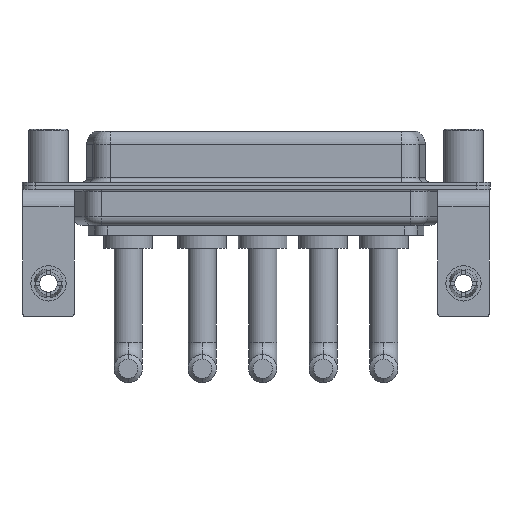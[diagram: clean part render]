
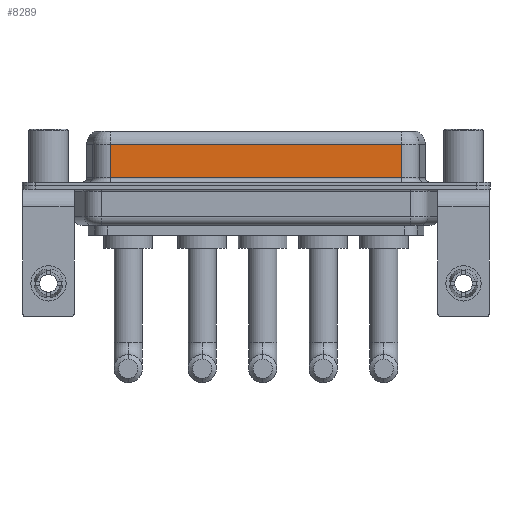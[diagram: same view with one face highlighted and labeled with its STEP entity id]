
A CAD part, front view. The second image highlights one B-rep face of the part: STEP entity #8289.
In plain terms, the highlighted planar face has unit normal (0, -1, 0).
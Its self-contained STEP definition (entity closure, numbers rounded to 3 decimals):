
#295 = VECTOR ( 'NONE', #5341, 1000. ) ;
#356 = CARTESIAN_POINT ( 'NONE',  ( 40.037, -3.95, 4.65 ) ) ;
#391 = PLANE ( 'NONE',  #2152 ) ;
#1579 = LINE ( 'NONE', #356, #295 ) ;
#1739 = ORIENTED_EDGE ( 'NONE', *, *, #10277, .T. ) ;
#2152 = AXIS2_PLACEMENT_3D ( 'NONE', #9179, #5371, #11518 ) ;
#2811 = CARTESIAN_POINT ( 'NONE',  ( 7.013, -3.95, 6.4 ) ) ;
#3545 = DIRECTION ( 'NONE',  ( 0., 0., -1. ) ) ;
#5341 = DIRECTION ( 'NONE',  ( -1., 0., 0. ) ) ;
#5371 = DIRECTION ( 'NONE',  ( 0., 1., 0. ) ) ;
#5410 = CARTESIAN_POINT ( 'NONE',  ( 40.037, -3.95, 0.9 ) ) ;
#5610 = VERTEX_POINT ( 'NONE', #8676 ) ;
#5750 = ORIENTED_EDGE ( 'NONE', *, *, #9745, .T. ) ;
#5841 = LINE ( 'NONE', #8318, #9047 ) ;
#6472 = VECTOR ( 'NONE', #12960, 1000. ) ;
#7248 = CARTESIAN_POINT ( 'NONE',  ( 7.013, -3.95, 0.9 ) ) ;
#7345 = VERTEX_POINT ( 'NONE', #7248 ) ;
#7417 = EDGE_CURVE ( 'NONE', #7345, #12870, #5841, .T. ) ;
#7426 = LINE ( 'NONE', #8497, #13387 ) ;
#7943 = ORIENTED_EDGE ( 'NONE', *, *, #7417, .T. ) ;
#7944 = FACE_OUTER_BOUND ( 'NONE', #11529, .T. ) ;
#8289 = ADVANCED_FACE ( 'NONE', ( #7944 ), #391, .F. ) ;
#8318 = CARTESIAN_POINT ( 'NONE',  ( 40.037, -3.95, 0.9 ) ) ;
#8497 = CARTESIAN_POINT ( 'NONE',  ( 40.037, -3.95, 6.4 ) ) ;
#8676 = CARTESIAN_POINT ( 'NONE',  ( 7.013, -3.95, 4.65 ) ) ;
#9047 = VECTOR ( 'NONE', #11063, 1000. ) ;
#9179 = CARTESIAN_POINT ( 'NONE',  ( 40.037, -3.95, 6.4 ) ) ;
#9745 = EDGE_CURVE ( 'NONE', #5610, #7345, #14123, .T. ) ;
#10277 = EDGE_CURVE ( 'NONE', #13058, #5610, #1579, .T. ) ;
#11063 = DIRECTION ( 'NONE',  ( 1., 0., 0. ) ) ;
#11518 = DIRECTION ( 'NONE',  ( 0., 0., 1. ) ) ;
#11529 = EDGE_LOOP ( 'NONE', ( #16095, #1739, #5750, #7943 ) ) ;
#12561 = EDGE_CURVE ( 'NONE', #13058, #12870, #7426, .T. ) ;
#12870 = VERTEX_POINT ( 'NONE', #5410 ) ;
#12960 = DIRECTION ( 'NONE',  ( 0., 0., -1. ) ) ;
#13058 = VERTEX_POINT ( 'NONE', #13531 ) ;
#13387 = VECTOR ( 'NONE', #3545, 1000. ) ;
#13531 = CARTESIAN_POINT ( 'NONE',  ( 40.037, -3.95, 4.65 ) ) ;
#14123 = LINE ( 'NONE', #2811, #6472 ) ;
#16095 = ORIENTED_EDGE ( 'NONE', *, *, #12561, .F. ) ;
